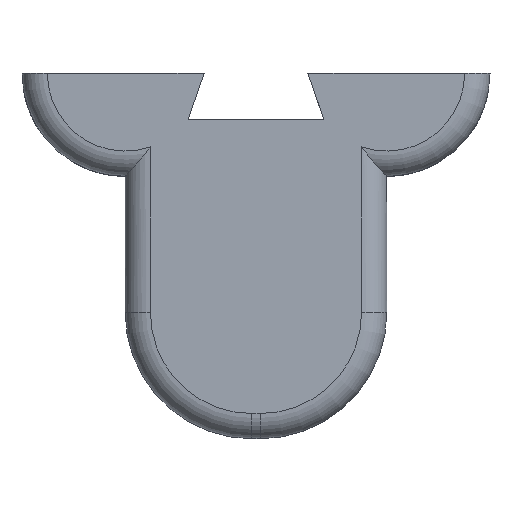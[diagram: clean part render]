
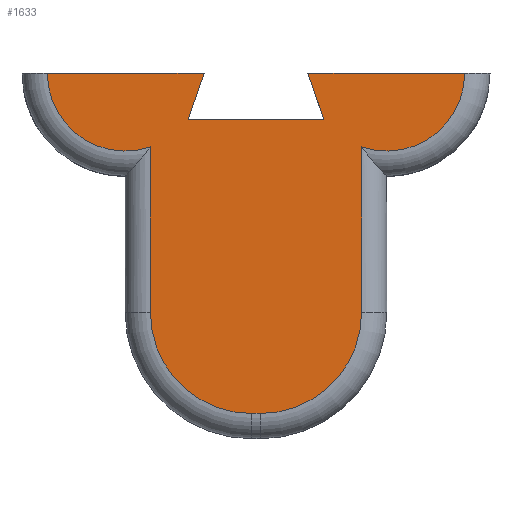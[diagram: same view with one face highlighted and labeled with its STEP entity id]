
A CAD part, front view. The second image highlights one B-rep face of the part: STEP entity #1633.
In plain terms, the highlighted planar face has unit normal (0, -1, 0).
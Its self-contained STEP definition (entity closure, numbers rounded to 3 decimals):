
#20=PLANE('',#1744);
#76=LINE('',#2945,#216);
#80=LINE('',#2953,#220);
#81=LINE('',#2955,#221);
#82=LINE('',#2957,#222);
#83=LINE('',#2958,#223);
#84=LINE('',#2960,#224);
#85=LINE('',#2964,#225);
#86=LINE('',#2967,#226);
#216=VECTOR('',#1903,10.);
#220=VECTOR('',#1909,10.);
#221=VECTOR('',#1910,10.);
#222=VECTOR('',#1911,10.);
#223=VECTOR('',#1912,10.);
#224=VECTOR('',#1913,10.);
#225=VECTOR('',#1916,10.);
#226=VECTOR('',#1919,10.);
#387=FACE_OUTER_BOUND('',#478,.T.);
#478=EDGE_LOOP('',(#1181,#1182,#1183,#1184,#1185,#1186,#1187,#1188,#1189,
#1190,#1191,#1192));
#650=CIRCLE('',#1735,6.15);
#655=CIRCLE('',#1742,6.15);
#656=CIRCLE('',#1745,8.);
#657=CIRCLE('',#1746,8.);
#680=VERTEX_POINT('',#2250);
#681=VERTEX_POINT('',#2252);
#744=VERTEX_POINT('',#2922);
#747=VERTEX_POINT('',#2927);
#748=VERTEX_POINT('',#2944);
#751=VERTEX_POINT('',#2952);
#752=VERTEX_POINT('',#2954);
#753=VERTEX_POINT('',#2956);
#754=VERTEX_POINT('',#2959);
#755=VERTEX_POINT('',#2961);
#756=VERTEX_POINT('',#2963);
#757=VERTEX_POINT('',#2965);
#848=EDGE_CURVE('',#680,#681,#650,.T.);
#916=EDGE_CURVE('',#747,#744,#655,.T.);
#917=EDGE_CURVE('',#744,#748,#76,.T.);
#921=EDGE_CURVE('',#751,#680,#80,.T.);
#922=EDGE_CURVE('',#751,#752,#81,.T.);
#923=EDGE_CURVE('',#752,#753,#82,.T.);
#924=EDGE_CURVE('',#753,#748,#83,.T.);
#925=EDGE_CURVE('',#754,#747,#84,.T.);
#926=EDGE_CURVE('',#755,#754,#656,.T.);
#927=EDGE_CURVE('',#756,#755,#85,.T.);
#928=EDGE_CURVE('',#757,#756,#657,.T.);
#929=EDGE_CURVE('',#681,#757,#86,.T.);
#1181=ORIENTED_EDGE('',*,*,#848,.F.);
#1182=ORIENTED_EDGE('',*,*,#921,.F.);
#1183=ORIENTED_EDGE('',*,*,#922,.T.);
#1184=ORIENTED_EDGE('',*,*,#923,.T.);
#1185=ORIENTED_EDGE('',*,*,#924,.T.);
#1186=ORIENTED_EDGE('',*,*,#917,.F.);
#1187=ORIENTED_EDGE('',*,*,#916,.F.);
#1188=ORIENTED_EDGE('',*,*,#925,.F.);
#1189=ORIENTED_EDGE('',*,*,#926,.F.);
#1190=ORIENTED_EDGE('',*,*,#927,.F.);
#1191=ORIENTED_EDGE('',*,*,#928,.F.);
#1192=ORIENTED_EDGE('',*,*,#929,.F.);
#1633=ADVANCED_FACE('',(#387),#20,.F.);
#1735=AXIS2_PLACEMENT_3D('',#2253,#1863,#1864);
#1742=AXIS2_PLACEMENT_3D('',#2942,#1899,#1900);
#1744=AXIS2_PLACEMENT_3D('',#2951,#1907,#1908);
#1745=AXIS2_PLACEMENT_3D('',#2962,#1914,#1915);
#1746=AXIS2_PLACEMENT_3D('',#2966,#1917,#1918);
#1863=DIRECTION('center_axis',(0.,1.,0.));
#1864=DIRECTION('ref_axis',(0.614,0.,-0.789));
#1899=DIRECTION('center_axis',(0.,1.,0.));
#1900=DIRECTION('ref_axis',(-0.614,0.,-0.789));
#1903=DIRECTION('',(1.,0.,0.));
#1907=DIRECTION('center_axis',(0.,1.,0.));
#1908=DIRECTION('ref_axis',(1.,0.,0.));
#1909=DIRECTION('',(1.,0.,0.));
#1910=DIRECTION('',(0.328,0.,-0.945));
#1911=DIRECTION('',(-1.,0.,0.));
#1912=DIRECTION('',(0.328,0.,0.945));
#1913=DIRECTION('',(0.,0.,1.));
#1914=DIRECTION('center_axis',(0.,1.,0.));
#1915=DIRECTION('ref_axis',(-0.707,0.,-0.707));
#1916=DIRECTION('',(-1.,0.,0.));
#1917=DIRECTION('center_axis',(0.,1.,0.));
#1918=DIRECTION('ref_axis',(0.707,0.,-0.707));
#1919=DIRECTION('',(0.,0.,-1.));
#2250=CARTESIAN_POINT('',(35.,0.,8.15));
#2252=CARTESIAN_POINT('',(26.85,0.,2.334));
#2253=CARTESIAN_POINT('Origin',(28.85,0.,8.15));
#2922=CARTESIAN_POINT('',(2.,0.,8.15));
#2927=CARTESIAN_POINT('',(10.15,0.,2.334));
#2942=CARTESIAN_POINT('Origin',(8.15,0.,8.15));
#2944=CARTESIAN_POINT('',(14.4,0.,8.15));
#2945=CARTESIAN_POINT('',(0.,0.,8.15));
#2951=CARTESIAN_POINT('Origin',(18.5,0.,4.075));
#2952=CARTESIAN_POINT('',(22.6,0.,8.15));
#2953=CARTESIAN_POINT('',(0.,0.,8.15));
#2954=CARTESIAN_POINT('',(23.875,0.,4.48));
#2955=CARTESIAN_POINT('',(23.011,0.,6.967));
#2956=CARTESIAN_POINT('',(13.125,0.,4.48));
#2957=CARTESIAN_POINT('',(21.188,0.,4.48));
#2958=CARTESIAN_POINT('',(13.352,0.,5.132));
#2959=CARTESIAN_POINT('',(10.15,0.,-10.75));
#2960=CARTESIAN_POINT('',(10.15,0.,-3.15));
#2961=CARTESIAN_POINT('',(18.15,0.,-18.75));
#2962=CARTESIAN_POINT('Origin',(18.15,0.,-10.75));
#2963=CARTESIAN_POINT('',(18.85,0.,-18.75));
#2964=CARTESIAN_POINT('',(18.5,0.,-18.75));
#2965=CARTESIAN_POINT('',(26.85,0.,-10.75));
#2966=CARTESIAN_POINT('Origin',(18.85,0.,-10.75));
#2967=CARTESIAN_POINT('',(26.85,0.,-3.15));
